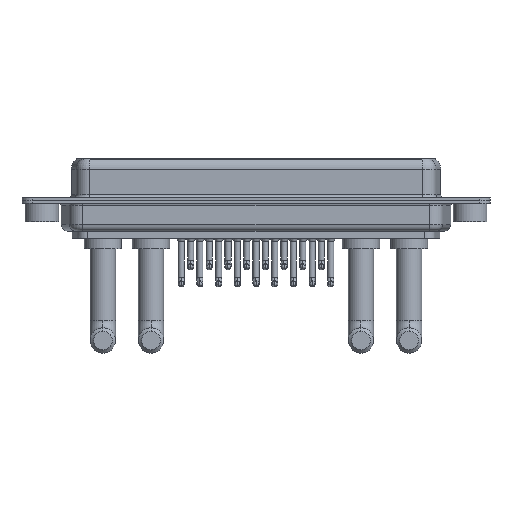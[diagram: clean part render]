
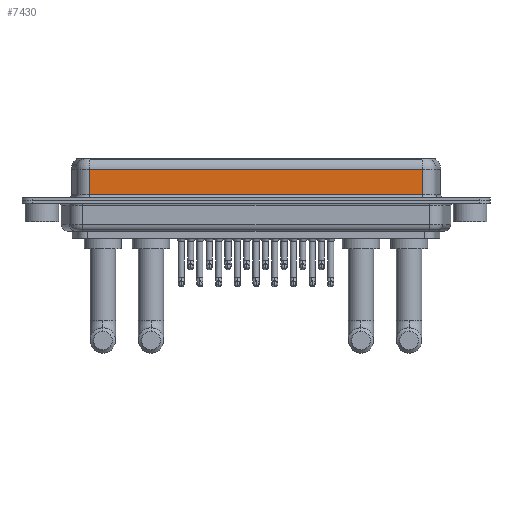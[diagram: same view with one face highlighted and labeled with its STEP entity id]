
A CAD part, front view. The second image highlights one B-rep face of the part: STEP entity #7430.
In plain terms, the highlighted planar face has unit normal (0, -1, 0).
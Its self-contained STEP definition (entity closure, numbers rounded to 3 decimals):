
#1025 = ORIENTED_EDGE ( 'NONE', *, *, #3376, .T. ) ;
#1084 = VECTOR ( 'NONE', #17389, 1000. ) ;
#1375 = PLANE ( 'NONE',  #8353 ) ;
#1762 = CARTESIAN_POINT ( 'NONE',  ( 7.038, -3.95, 6.4 ) ) ;
#2240 = CARTESIAN_POINT ( 'NONE',  ( 56.462, -3.95, 0.9 ) ) ;
#2538 = CARTESIAN_POINT ( 'NONE',  ( 7.038, -3.95, 0.9 ) ) ;
#3376 = EDGE_CURVE ( 'NONE', #17664, #20449, #15495, .T. ) ;
#3426 = CARTESIAN_POINT ( 'NONE',  ( 56.462, -3.95, 0.9 ) ) ;
#3438 = LINE ( 'NONE', #1762, #13870 ) ;
#3744 = CARTESIAN_POINT ( 'NONE',  ( 56.462, -3.95, 6.4 ) ) ;
#3756 = CARTESIAN_POINT ( 'NONE',  ( 56.462, -3.95, 4.65 ) ) ;
#6612 = DIRECTION ( 'NONE',  ( 0., 1., 0. ) ) ;
#7022 = VERTEX_POINT ( 'NONE', #2538 ) ;
#7198 = LINE ( 'NONE', #3744, #15371 ) ;
#7430 = ADVANCED_FACE ( 'NONE', ( #21890 ), #1375, .F. ) ;
#7932 = ORIENTED_EDGE ( 'NONE', *, *, #13335, .F. ) ;
#8181 = CARTESIAN_POINT ( 'NONE',  ( 56.462, -3.95, 6.4 ) ) ;
#8353 = AXIS2_PLACEMENT_3D ( 'NONE', #8181, #6612, #13430 ) ;
#8581 = DIRECTION ( 'NONE',  ( 0., 0., -1. ) ) ;
#8855 = ORIENTED_EDGE ( 'NONE', *, *, #20887, .T. ) ;
#9723 = ORIENTED_EDGE ( 'NONE', *, *, #10282, .T. ) ;
#10282 = EDGE_CURVE ( 'NONE', #7022, #19624, #20981, .T. ) ;
#10568 = DIRECTION ( 'NONE',  ( 0., 0., -1. ) ) ;
#11196 = DIRECTION ( 'NONE',  ( 1., 0., 0. ) ) ;
#12949 = CARTESIAN_POINT ( 'NONE',  ( 7.038, -3.95, 4.65 ) ) ;
#13335 = EDGE_CURVE ( 'NONE', #17664, #19624, #7198, .T. ) ;
#13430 = DIRECTION ( 'NONE',  ( 0., 0., 1. ) ) ;
#13870 = VECTOR ( 'NONE', #8581, 1000. ) ;
#15371 = VECTOR ( 'NONE', #10568, 1000. ) ;
#15495 = LINE ( 'NONE', #3756, #1084 ) ;
#15627 = EDGE_LOOP ( 'NONE', ( #7932, #1025, #8855, #9723 ) ) ;
#16719 = CARTESIAN_POINT ( 'NONE',  ( 56.462, -3.95, 4.65 ) ) ;
#17389 = DIRECTION ( 'NONE',  ( -1., 0., 0. ) ) ;
#17664 = VERTEX_POINT ( 'NONE', #16719 ) ;
#19624 = VERTEX_POINT ( 'NONE', #3426 ) ;
#20449 = VERTEX_POINT ( 'NONE', #12949 ) ;
#20887 = EDGE_CURVE ( 'NONE', #20449, #7022, #3438, .T. ) ;
#20981 = LINE ( 'NONE', #2240, #22066 ) ;
#21890 = FACE_OUTER_BOUND ( 'NONE', #15627, .T. ) ;
#22066 = VECTOR ( 'NONE', #11196, 1000. ) ;
